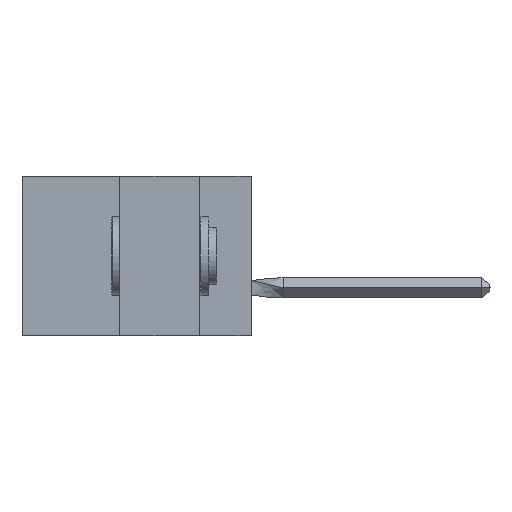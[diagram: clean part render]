
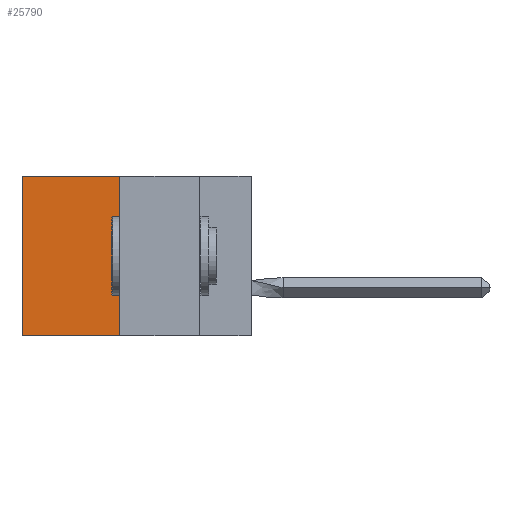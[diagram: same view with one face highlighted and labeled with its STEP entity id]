
A CAD part, left-side view. The second image highlights one B-rep face of the part: STEP entity #25790.
In plain terms, the highlighted planar face has unit normal (-1, 0, 0).
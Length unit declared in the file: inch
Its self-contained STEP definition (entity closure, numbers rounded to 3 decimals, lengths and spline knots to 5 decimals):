
#562 = CARTESIAN_POINT ( 'NONE',  ( 0.305, 0.413, -0.5 ) ) ;
#646 = FACE_OUTER_BOUND ( 'NONE', #25718, .T. ) ;
#3572 = DIRECTION ( 'NONE',  ( 0., 0., -1. ) ) ;
#4666 = AXIS2_PLACEMENT_3D ( 'NONE', #562, #24809, #8684 ) ;
#4888 = CARTESIAN_POINT ( 'NONE',  ( 0.305, 0.413, 0. ) ) ;
#6376 = DIRECTION ( 'NONE',  ( 0., 1., 0. ) ) ;
#7484 = VECTOR ( 'NONE', #6376, 39.37008 ) ;
#7940 = DIRECTION ( 'NONE',  ( 0., 1., 0. ) ) ;
#8248 = VERTEX_POINT ( 'NONE', #19217 ) ;
#8684 = DIRECTION ( 'NONE',  ( 0., 0., -1. ) ) ;
#8752 = ORIENTED_EDGE ( 'NONE', *, *, #23384, .F. ) ;
#11199 = LINE ( 'NONE', #18348, #28021 ) ;
#11818 = EDGE_CURVE ( 'NONE', #26171, #15102, #11199, .T. ) ;
#13642 = VERTEX_POINT ( 'NONE', #19742 ) ;
#15102 = VERTEX_POINT ( 'NONE', #26305 ) ;
#15170 = VECTOR ( 'NONE', #3572, 39.37008 ) ;
#15455 = ORIENTED_EDGE ( 'NONE', *, *, #29410, .T. ) ;
#18348 = CARTESIAN_POINT ( 'NONE',  ( 0.305, 0.72, -0.5 ) ) ;
#18378 = ORIENTED_EDGE ( 'NONE', *, *, #11818, .T. ) ;
#18525 = VECTOR ( 'NONE', #7940, 39.37008 ) ;
#19217 = CARTESIAN_POINT ( 'NONE',  ( 0.305, 0.413, 0. ) ) ;
#19742 = CARTESIAN_POINT ( 'NONE',  ( 0.305, 0.413, -0.5 ) ) ;
#21534 = ORIENTED_EDGE ( 'NONE', *, *, #24762, .F. ) ;
#22615 = CARTESIAN_POINT ( 'NONE',  ( 0.305, 0.413, -0.5 ) ) ;
#23384 = EDGE_CURVE ( 'NONE', #8248, #13642, #32425, .T. ) ;
#23572 = CARTESIAN_POINT ( 'NONE',  ( 0.305, 0.72, 0. ) ) ;
#24762 = EDGE_CURVE ( 'NONE', #13642, #15102, #31007, .T. ) ;
#24809 = DIRECTION ( 'NONE',  ( 1., 0., 0. ) ) ;
#25718 = EDGE_LOOP ( 'NONE', ( #18378, #21534, #8752, #15455 ) ) ;
#25790 = ADVANCED_FACE ( 'NONE', ( #646 ), #32845, .F. ) ;
#26171 = VERTEX_POINT ( 'NONE', #23572 ) ;
#26305 = CARTESIAN_POINT ( 'NONE',  ( 0.305, 0.72, -0.5 ) ) ;
#26477 = DIRECTION ( 'NONE',  ( 0., 0., -1. ) ) ;
#28021 = VECTOR ( 'NONE', #26477, 39.37008 ) ;
#29410 = EDGE_CURVE ( 'NONE', #8248, #26171, #29858, .T. ) ;
#29858 = LINE ( 'NONE', #4888, #18525 ) ;
#30585 = CARTESIAN_POINT ( 'NONE',  ( 0.305, 0.413, -0.5 ) ) ;
#31007 = LINE ( 'NONE', #22615, #7484 ) ;
#32425 = LINE ( 'NONE', #30585, #15170 ) ;
#32845 = PLANE ( 'NONE',  #4666 ) ;
